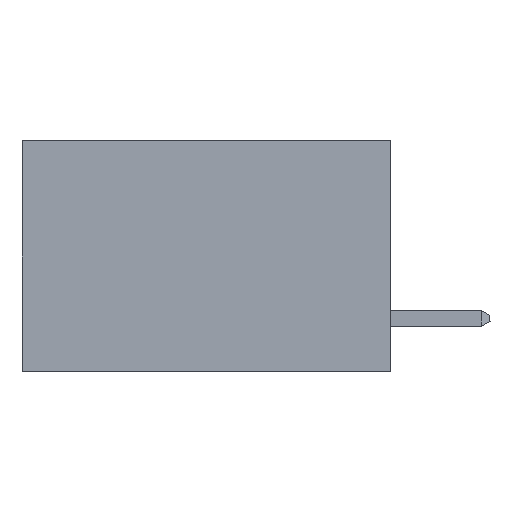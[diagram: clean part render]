
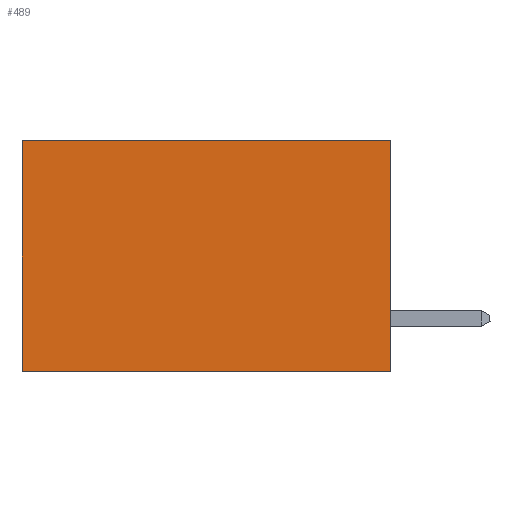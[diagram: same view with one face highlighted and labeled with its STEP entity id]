
A CAD part, left-side view. The second image highlights one B-rep face of the part: STEP entity #489.
In plain terms, the highlighted planar face has unit normal (-1, 0, 0).
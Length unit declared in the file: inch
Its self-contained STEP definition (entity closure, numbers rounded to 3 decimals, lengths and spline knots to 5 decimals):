
#322 = PLANE ( 'NONE',  #11722 ) ;
#489 = ADVANCED_FACE ( 'NONE', ( #1184 ), #322, .F. ) ;
#790 = ORIENTED_EDGE ( 'NONE', *, *, #6252, .T. ) ;
#859 = ORIENTED_EDGE ( 'NONE', *, *, #1528, .F. ) ;
#903 = CARTESIAN_POINT ( 'NONE',  ( 0.277, 0., -0.37 ) ) ;
#909 = ORIENTED_EDGE ( 'NONE', *, *, #14882, .F. ) ;
#999 = ORIENTED_EDGE ( 'NONE', *, *, #9998, .T. ) ;
#1184 = FACE_OUTER_BOUND ( 'NONE', #11796, .T. ) ;
#1528 = EDGE_CURVE ( 'NONE', #15142, #13002, #5678, .T. ) ;
#2535 = DIRECTION ( 'NONE',  ( 0., 1., 0. ) ) ;
#3886 = CARTESIAN_POINT ( 'NONE',  ( 0.277, 0., -0.37 ) ) ;
#5031 = VERTEX_POINT ( 'NONE', #11334 ) ;
#5268 = CARTESIAN_POINT ( 'NONE',  ( 0.277, 0., 0. ) ) ;
#5678 = LINE ( 'NONE', #10942, #11972 ) ;
#6252 = EDGE_CURVE ( 'NONE', #5031, #13002, #9368, .T. ) ;
#6513 = VERTEX_POINT ( 'NONE', #5268 ) ;
#7129 = CARTESIAN_POINT ( 'NONE',  ( 0.277, 0., -0.37 ) ) ;
#7410 = VECTOR ( 'NONE', #10676, 39.37008 ) ;
#8704 = DIRECTION ( 'NONE',  ( 0., 0., -1. ) ) ;
#8758 = CARTESIAN_POINT ( 'NONE',  ( 0.277, 0.59, -0.37 ) ) ;
#9315 = DIRECTION ( 'NONE',  ( 0., 1., 0. ) ) ;
#9368 = LINE ( 'NONE', #8758, #14154 ) ;
#9998 = EDGE_CURVE ( 'NONE', #6513, #5031, #14745, .T. ) ;
#10165 = LINE ( 'NONE', #7129, #7410 ) ;
#10676 = DIRECTION ( 'NONE',  ( 0., 0., -1. ) ) ;
#10921 = CARTESIAN_POINT ( 'NONE',  ( 0.277, 0., 0. ) ) ;
#10942 = CARTESIAN_POINT ( 'NONE',  ( 0.277, 0., -0.37 ) ) ;
#11018 = DIRECTION ( 'NONE',  ( 1., 0., 0. ) ) ;
#11334 = CARTESIAN_POINT ( 'NONE',  ( 0.277, 0.59, 0. ) ) ;
#11533 = DIRECTION ( 'NONE',  ( 0., 0., -1. ) ) ;
#11682 = CARTESIAN_POINT ( 'NONE',  ( 0.277, 0.59, -0.37 ) ) ;
#11722 = AXIS2_PLACEMENT_3D ( 'NONE', #903, #11018, #11533 ) ;
#11796 = EDGE_LOOP ( 'NONE', ( #790, #859, #909, #999 ) ) ;
#11972 = VECTOR ( 'NONE', #9315, 39.37008 ) ;
#13002 = VERTEX_POINT ( 'NONE', #11682 ) ;
#14090 = VECTOR ( 'NONE', #2535, 39.37008 ) ;
#14154 = VECTOR ( 'NONE', #8704, 39.37008 ) ;
#14745 = LINE ( 'NONE', #10921, #14090 ) ;
#14882 = EDGE_CURVE ( 'NONE', #6513, #15142, #10165, .T. ) ;
#15142 = VERTEX_POINT ( 'NONE', #3886 ) ;
